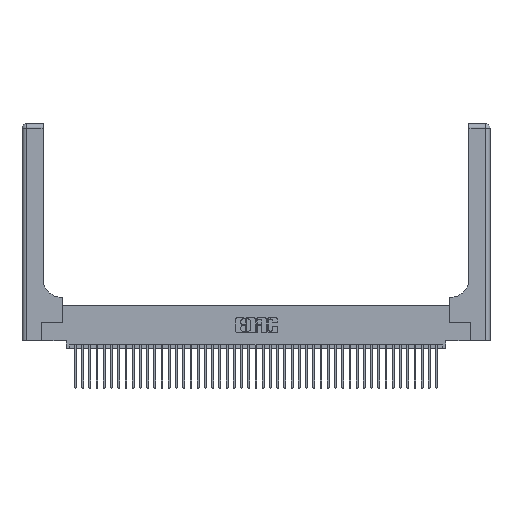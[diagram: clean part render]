
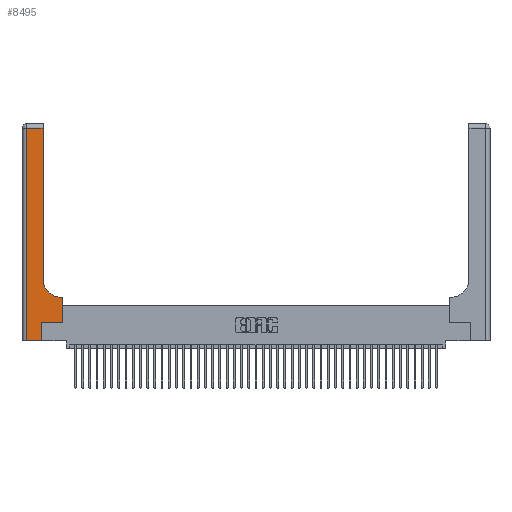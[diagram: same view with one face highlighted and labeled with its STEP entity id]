
A CAD part, top view. The second image highlights one B-rep face of the part: STEP entity #8495.
In plain terms, the highlighted planar face has unit normal (0, 0, 1).
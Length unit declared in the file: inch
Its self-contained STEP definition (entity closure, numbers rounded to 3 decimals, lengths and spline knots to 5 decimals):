
#807 = CARTESIAN_POINT ( 'NONE',  ( 0.2915, 2.94, 0.37 ) ) ;
#942 = CARTESIAN_POINT ( 'NONE',  ( 0.5585, 0.25, 0.37 ) ) ;
#1503 = EDGE_CURVE ( 'NONE', #43293, #20913, #23217, .T. ) ;
#1587 = VECTOR ( 'NONE', #36530, 39.37008 ) ;
#1686 = VERTEX_POINT ( 'NONE', #29450 ) ;
#2638 = ORIENTED_EDGE ( 'NONE', *, *, #1503, .T. ) ;
#2741 = VERTEX_POINT ( 'NONE', #26817 ) ;
#4421 = VERTEX_POINT ( 'NONE', #11410 ) ;
#4617 = DIRECTION ( 'NONE',  ( 0., 1., 0. ) ) ;
#4673 = LINE ( 'NONE', #34556, #11783 ) ;
#4789 = CARTESIAN_POINT ( 'NONE',  ( 0.06, 2.94, 0.37 ) ) ;
#4949 = CARTESIAN_POINT ( 'NONE',  ( 0.2915, 0.6, 0.37 ) ) ;
#5338 = EDGE_LOOP ( 'NONE', ( #43414, #15370, #20683, #39117, #11253, #31982, #6728, #2638, #34579 ) ) ;
#6301 = CARTESIAN_POINT ( 'NONE',  ( 0., 0., 0.37 ) ) ;
#6632 = VECTOR ( 'NONE', #9411, 39.37008 ) ;
#6728 = ORIENTED_EDGE ( 'NONE', *, *, #30905, .T. ) ;
#7719 = AXIS2_PLACEMENT_3D ( 'NONE', #24684, #30323, #28231 ) ;
#7989 = EDGE_CURVE ( 'NONE', #2741, #4421, #24617, .T. ) ;
#8495 = ADVANCED_FACE ( 'NONE', ( #27248 ), #33881, .F. ) ;
#8939 = LINE ( 'NONE', #26480, #29802 ) ;
#9411 = DIRECTION ( 'NONE',  ( -1., 0., 0. ) ) ;
#9421 = LINE ( 'NONE', #942, #15902 ) ;
#9432 = LINE ( 'NONE', #9851, #28116 ) ;
#9851 = CARTESIAN_POINT ( 'NONE',  ( 0.269, 0.25, 0.37 ) ) ;
#10012 = CARTESIAN_POINT ( 'NONE',  ( 0.5415, 0.85, 0.37 ) ) ;
#11253 = ORIENTED_EDGE ( 'NONE', *, *, #43053, .T. ) ;
#11410 = CARTESIAN_POINT ( 'NONE',  ( 0.269, 0., 0.37 ) ) ;
#11783 = VECTOR ( 'NONE', #14608, 39.37008 ) ;
#14586 = EDGE_CURVE ( 'NONE', #21251, #2741, #8939, .T. ) ;
#14608 = DIRECTION ( 'NONE',  ( 0., 1., 0. ) ) ;
#15370 = ORIENTED_EDGE ( 'NONE', *, *, #40557, .T. ) ;
#15698 = LINE ( 'NONE', #23100, #16831 ) ;
#15902 = VECTOR ( 'NONE', #4617, 39.37008 ) ;
#16126 = EDGE_CURVE ( 'NONE', #26032, #1686, #9432, .T. ) ;
#16658 = DIRECTION ( 'NONE',  ( 0., 0., -1. ) ) ;
#16793 = DIRECTION ( 'NONE',  ( 1., 0., 0. ) ) ;
#16831 = VECTOR ( 'NONE', #33650, 39.37008 ) ;
#16833 = DIRECTION ( 'NONE',  ( 1., 0., 0. ) ) ;
#17470 = VERTEX_POINT ( 'NONE', #37728 ) ;
#19675 = EDGE_CURVE ( 'NONE', #20913, #17470, #34599, .T. ) ;
#19727 = LINE ( 'NONE', #42951, #1587 ) ;
#20352 = AXIS2_PLACEMENT_3D ( 'NONE', #10012, #16658, #23624 ) ;
#20683 = ORIENTED_EDGE ( 'NONE', *, *, #14586, .T. ) ;
#20913 = VERTEX_POINT ( 'NONE', #43914 ) ;
#21251 = VERTEX_POINT ( 'NONE', #4789 ) ;
#21998 = VERTEX_POINT ( 'NONE', #807 ) ;
#22748 = EDGE_CURVE ( 'NONE', #17470, #21998, #15698, .T. ) ;
#23100 = CARTESIAN_POINT ( 'NONE',  ( 0.2915, 3., 0.37 ) ) ;
#23217 = LINE ( 'NONE', #4949, #6632 ) ;
#23624 = DIRECTION ( 'NONE',  ( 1., 0., 0. ) ) ;
#24617 = LINE ( 'NONE', #6301, #33604 ) ;
#24684 = CARTESIAN_POINT ( 'NONE',  ( 0., 3., 0.37 ) ) ;
#26032 = VERTEX_POINT ( 'NONE', #27822 ) ;
#26480 = CARTESIAN_POINT ( 'NONE',  ( 0.06, 3., 0.37 ) ) ;
#26817 = CARTESIAN_POINT ( 'NONE',  ( 0.06, 0., 0.37 ) ) ;
#27248 = FACE_OUTER_BOUND ( 'NONE', #5338, .T. ) ;
#27822 = CARTESIAN_POINT ( 'NONE',  ( 0.269, 0.25, 0.37 ) ) ;
#28116 = VECTOR ( 'NONE', #16793, 39.37008 ) ;
#28231 = DIRECTION ( 'NONE',  ( -1., 0., 0. ) ) ;
#29450 = CARTESIAN_POINT ( 'NONE',  ( 0.5585, 0.25, 0.37 ) ) ;
#29802 = VECTOR ( 'NONE', #43481, 39.37008 ) ;
#30323 = DIRECTION ( 'NONE',  ( 0., 0., -1. ) ) ;
#30905 = EDGE_CURVE ( 'NONE', #1686, #43293, #9421, .T. ) ;
#31982 = ORIENTED_EDGE ( 'NONE', *, *, #16126, .T. ) ;
#33604 = VECTOR ( 'NONE', #16833, 39.37008 ) ;
#33650 = DIRECTION ( 'NONE',  ( 0., 1., 0. ) ) ;
#33881 = PLANE ( 'NONE',  #7719 ) ;
#34556 = CARTESIAN_POINT ( 'NONE',  ( 0.269, 0., 0.37 ) ) ;
#34579 = ORIENTED_EDGE ( 'NONE', *, *, #19675, .T. ) ;
#34599 = CIRCLE ( 'NONE', #20352, 0.25 ) ;
#36530 = DIRECTION ( 'NONE',  ( -1., 0., 0. ) ) ;
#37728 = CARTESIAN_POINT ( 'NONE',  ( 0.2915, 0.85, 0.37 ) ) ;
#39117 = ORIENTED_EDGE ( 'NONE', *, *, #7989, .T. ) ;
#40084 = CARTESIAN_POINT ( 'NONE',  ( 0.5585, 0.6, 0.37 ) ) ;
#40557 = EDGE_CURVE ( 'NONE', #21998, #21251, #19727, .T. ) ;
#42951 = CARTESIAN_POINT ( 'NONE',  ( 0., 2.94, 0.37 ) ) ;
#43053 = EDGE_CURVE ( 'NONE', #4421, #26032, #4673, .T. ) ;
#43293 = VERTEX_POINT ( 'NONE', #40084 ) ;
#43414 = ORIENTED_EDGE ( 'NONE', *, *, #22748, .T. ) ;
#43481 = DIRECTION ( 'NONE',  ( 0., -1., 0. ) ) ;
#43914 = CARTESIAN_POINT ( 'NONE',  ( 0.5415, 0.6, 0.37 ) ) ;
